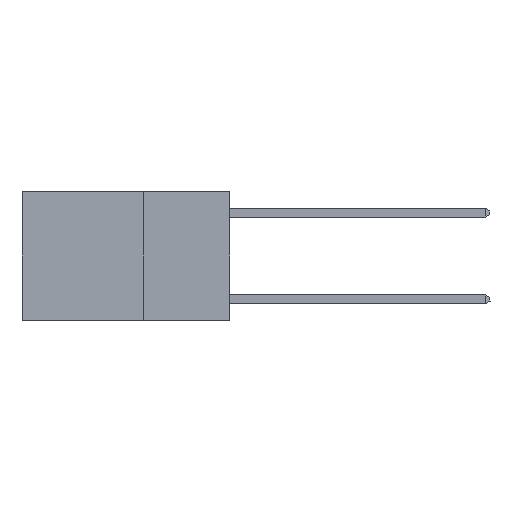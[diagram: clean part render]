
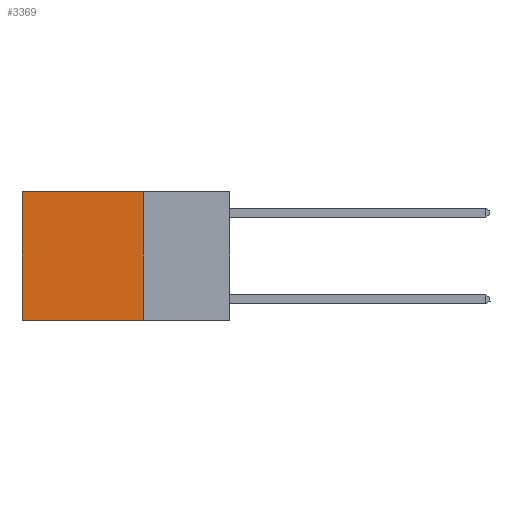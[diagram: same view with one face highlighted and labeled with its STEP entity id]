
A CAD part, left-side view. The second image highlights one B-rep face of the part: STEP entity #3369.
In plain terms, the highlighted planar face has unit normal (-1, 0, 0).
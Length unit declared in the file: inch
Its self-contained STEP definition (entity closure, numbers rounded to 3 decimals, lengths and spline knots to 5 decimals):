
#201 = VERTEX_POINT ( 'NONE', #10256 ) ;
#575 = EDGE_CURVE ( 'NONE', #5448, #201, #23535, .T. ) ;
#1281 = EDGE_CURVE ( 'NONE', #8417, #10713, #13179, .T. ) ;
#1895 = VECTOR ( 'NONE', #5516, 39.37008 ) ;
#2519 = DIRECTION ( 'NONE',  ( 0., 1., 0. ) ) ;
#2912 = CARTESIAN_POINT ( 'NONE',  ( 0.2625, 0.25, 0. ) ) ;
#3089 = CARTESIAN_POINT ( 'NONE',  ( 0.2625, 0.6, -0.37 ) ) ;
#3369 = ADVANCED_FACE ( 'NONE', ( #10980 ), #16926, .F. ) ;
#3426 = CARTESIAN_POINT ( 'NONE',  ( 0.2625, 0.25, 0. ) ) ;
#4688 = LINE ( 'NONE', #13536, #9386 ) ;
#4965 = DIRECTION ( 'NONE',  ( 1., 0., 0. ) ) ;
#5448 = VERTEX_POINT ( 'NONE', #14200 ) ;
#5516 = DIRECTION ( 'NONE',  ( 0., 0., -1. ) ) ;
#7487 = ORIENTED_EDGE ( 'NONE', *, *, #14022, .T. ) ;
#7597 = ORIENTED_EDGE ( 'NONE', *, *, #17292, .F. ) ;
#8227 = VECTOR ( 'NONE', #9291, 39.37008 ) ;
#8417 = VERTEX_POINT ( 'NONE', #9036 ) ;
#9036 = CARTESIAN_POINT ( 'NONE',  ( 0.2625, 0.6, 0. ) ) ;
#9291 = DIRECTION ( 'NONE',  ( 0., 0., -1. ) ) ;
#9386 = VECTOR ( 'NONE', #9623, 39.37008 ) ;
#9623 = DIRECTION ( 'NONE',  ( 0., 1., 0. ) ) ;
#10256 = CARTESIAN_POINT ( 'NONE',  ( 0.2625, 0.25, -0.37 ) ) ;
#10713 = VERTEX_POINT ( 'NONE', #3089 ) ;
#10980 = FACE_OUTER_BOUND ( 'NONE', #14687, .T. ) ;
#13179 = LINE ( 'NONE', #25356, #1895 ) ;
#13536 = CARTESIAN_POINT ( 'NONE',  ( 0.2625, 0.25, 0. ) ) ;
#14022 = EDGE_CURVE ( 'NONE', #5448, #8417, #4688, .T. ) ;
#14061 = AXIS2_PLACEMENT_3D ( 'NONE', #2912, #4965, #18927 ) ;
#14200 = CARTESIAN_POINT ( 'NONE',  ( 0.2625, 0.25, 0. ) ) ;
#14556 = VECTOR ( 'NONE', #2519, 39.37008 ) ;
#14687 = EDGE_LOOP ( 'NONE', ( #15822, #7597, #19566, #7487 ) ) ;
#15822 = ORIENTED_EDGE ( 'NONE', *, *, #1281, .T. ) ;
#16523 = CARTESIAN_POINT ( 'NONE',  ( 0.2625, 0.25, -0.37 ) ) ;
#16926 = PLANE ( 'NONE',  #14061 ) ;
#17292 = EDGE_CURVE ( 'NONE', #201, #10713, #19887, .T. ) ;
#18927 = DIRECTION ( 'NONE',  ( 0., 0., -1. ) ) ;
#19566 = ORIENTED_EDGE ( 'NONE', *, *, #575, .F. ) ;
#19887 = LINE ( 'NONE', #16523, #14556 ) ;
#23535 = LINE ( 'NONE', #3426, #8227 ) ;
#25356 = CARTESIAN_POINT ( 'NONE',  ( 0.2625, 0.6, 0. ) ) ;
